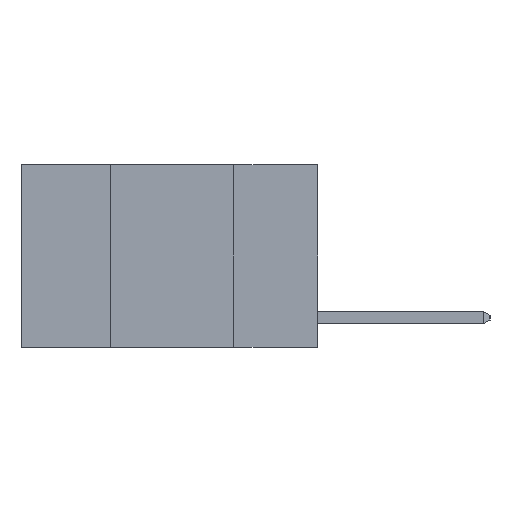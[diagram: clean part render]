
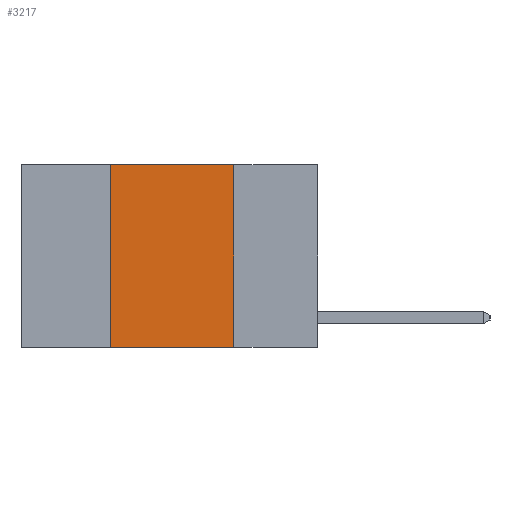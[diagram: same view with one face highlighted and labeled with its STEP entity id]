
A CAD part, left-side view. The second image highlights one B-rep face of the part: STEP entity #3217.
In plain terms, the highlighted planar face has unit normal (-1, 0, 0).
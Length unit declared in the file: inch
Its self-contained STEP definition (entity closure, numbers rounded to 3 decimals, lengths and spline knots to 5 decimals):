
#76 = ORIENTED_EDGE ( 'NONE', *, *, #9357, .F. ) ;
#581 = VERTEX_POINT ( 'NONE', #6636 ) ;
#629 = FACE_OUTER_BOUND ( 'NONE', #11009, .T. ) ;
#2079 = VERTEX_POINT ( 'NONE', #8854 ) ;
#2084 = ORIENTED_EDGE ( 'NONE', *, *, #7036, .F. ) ;
#2154 = EDGE_CURVE ( 'NONE', #4238, #10549, #4909, .T. ) ;
#2664 = VECTOR ( 'NONE', #3576, 39.37008 ) ;
#2694 = DIRECTION ( 'NONE',  ( 0., 0., 1. ) ) ;
#3120 = VECTOR ( 'NONE', #10029, 39.37008 ) ;
#3154 = CARTESIAN_POINT ( 'NONE',  ( 0., 0.6, 0. ) ) ;
#3217 = ADVANCED_FACE ( 'NONE', ( #629 ), #4824, .F. ) ;
#3554 = CARTESIAN_POINT ( 'NONE',  ( 0., 0.42, 0. ) ) ;
#3576 = DIRECTION ( 'NONE',  ( 0., 0., -1. ) ) ;
#4238 = VERTEX_POINT ( 'NONE', #6389 ) ;
#4599 = CARTESIAN_POINT ( 'NONE',  ( 0., 0.17, -0.37 ) ) ;
#4824 = PLANE ( 'NONE',  #6489 ) ;
#4909 = LINE ( 'NONE', #5828, #2664 ) ;
#5165 = DIRECTION ( 'NONE',  ( 0., 0., -1. ) ) ;
#5349 = LINE ( 'NONE', #3154, #3120 ) ;
#5828 = CARTESIAN_POINT ( 'NONE',  ( 0., 0.17, 0. ) ) ;
#6272 = VECTOR ( 'NONE', #2694, 39.37008 ) ;
#6363 = CARTESIAN_POINT ( 'NONE',  ( 0., 0.6, 0. ) ) ;
#6389 = CARTESIAN_POINT ( 'NONE',  ( 0., 0.17, 0. ) ) ;
#6489 = AXIS2_PLACEMENT_3D ( 'NONE', #6363, #7329, #5165 ) ;
#6559 = CARTESIAN_POINT ( 'NONE',  ( 0., 0.6, -0.37 ) ) ;
#6636 = CARTESIAN_POINT ( 'NONE',  ( 0., 0.42, -0.37 ) ) ;
#6840 = LINE ( 'NONE', #6559, #8584 ) ;
#7036 = EDGE_CURVE ( 'NONE', #2079, #4238, #5349, .T. ) ;
#7329 = DIRECTION ( 'NONE',  ( 1., 0., 0. ) ) ;
#8343 = EDGE_CURVE ( 'NONE', #581, #10549, #6840, .T. ) ;
#8561 = LINE ( 'NONE', #3554, #6272 ) ;
#8584 = VECTOR ( 'NONE', #10883, 39.37008 ) ;
#8854 = CARTESIAN_POINT ( 'NONE',  ( 0., 0.42, 0. ) ) ;
#9167 = ORIENTED_EDGE ( 'NONE', *, *, #8343, .T. ) ;
#9357 = EDGE_CURVE ( 'NONE', #581, #2079, #8561, .T. ) ;
#10029 = DIRECTION ( 'NONE',  ( 0., -1., 0. ) ) ;
#10549 = VERTEX_POINT ( 'NONE', #4599 ) ;
#10883 = DIRECTION ( 'NONE',  ( 0., -1., 0. ) ) ;
#10982 = ORIENTED_EDGE ( 'NONE', *, *, #2154, .F. ) ;
#11009 = EDGE_LOOP ( 'NONE', ( #10982, #2084, #76, #9167 ) ) ;
